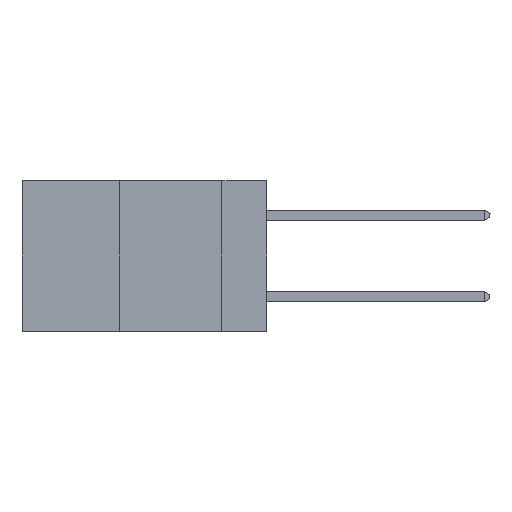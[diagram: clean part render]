
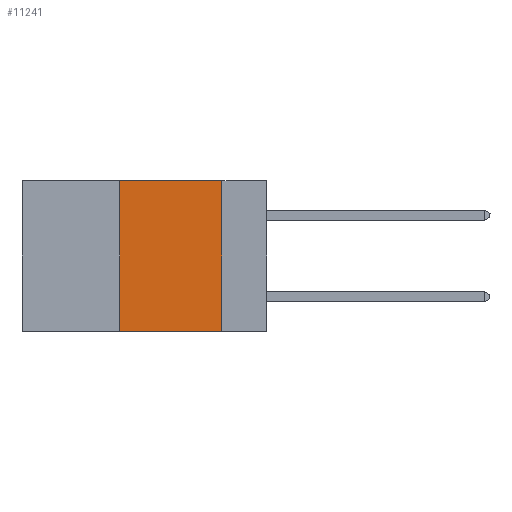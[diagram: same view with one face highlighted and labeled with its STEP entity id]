
A CAD part, left-side view. The second image highlights one B-rep face of the part: STEP entity #11241.
In plain terms, the highlighted planar face has unit normal (-1, 0, 0).
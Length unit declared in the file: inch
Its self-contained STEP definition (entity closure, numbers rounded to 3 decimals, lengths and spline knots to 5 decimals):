
#434 = LINE ( 'NONE', #5004, #16447 ) ;
#929 = EDGE_CURVE ( 'NONE', #17560, #944, #16275, .T. ) ;
#944 = VERTEX_POINT ( 'NONE', #15365 ) ;
#1764 = EDGE_LOOP ( 'NONE', ( #7990, #14603, #2605, #5064 ) ) ;
#2605 = ORIENTED_EDGE ( 'NONE', *, *, #18100, .F. ) ;
#3292 = LINE ( 'NONE', #14685, #11626 ) ;
#3982 = CARTESIAN_POINT ( 'NONE',  ( 0., 0.11, -0.37 ) ) ;
#4413 = AXIS2_PLACEMENT_3D ( 'NONE', #14234, #12730, #7152 ) ;
#5004 = CARTESIAN_POINT ( 'NONE',  ( 0., 0.6, -0.37 ) ) ;
#5064 = ORIENTED_EDGE ( 'NONE', *, *, #7106, .T. ) ;
#5637 = VERTEX_POINT ( 'NONE', #3982 ) ;
#7045 = EDGE_CURVE ( 'NONE', #944, #5637, #3292, .T. ) ;
#7106 = EDGE_CURVE ( 'NONE', #15491, #5637, #434, .T. ) ;
#7152 = DIRECTION ( 'NONE',  ( 0., 0., -1. ) ) ;
#7990 = ORIENTED_EDGE ( 'NONE', *, *, #7045, .F. ) ;
#8467 = FACE_OUTER_BOUND ( 'NONE', #1764, .T. ) ;
#8521 = DIRECTION ( 'NONE',  ( 0., -1., 0. ) ) ;
#9113 = DIRECTION ( 'NONE',  ( 0., -1., 0. ) ) ;
#9523 = CARTESIAN_POINT ( 'NONE',  ( 0., 0.36, -0.37 ) ) ;
#11241 = ADVANCED_FACE ( 'NONE', ( #8467 ), #15675, .F. ) ;
#11626 = VECTOR ( 'NONE', #11979, 39.37008 ) ;
#11979 = DIRECTION ( 'NONE',  ( 0., 0., -1. ) ) ;
#12608 = CARTESIAN_POINT ( 'NONE',  ( 0., 0.6, 0. ) ) ;
#12730 = DIRECTION ( 'NONE',  ( 1., 0., 0. ) ) ;
#13439 = CARTESIAN_POINT ( 'NONE',  ( 0., 0.36, 0. ) ) ;
#14229 = VECTOR ( 'NONE', #16125, 39.37008 ) ;
#14234 = CARTESIAN_POINT ( 'NONE',  ( 0., 0.6, 0. ) ) ;
#14603 = ORIENTED_EDGE ( 'NONE', *, *, #929, .F. ) ;
#14685 = CARTESIAN_POINT ( 'NONE',  ( 0., 0.11, 0. ) ) ;
#14748 = CARTESIAN_POINT ( 'NONE',  ( 0., 0.36, 0. ) ) ;
#15365 = CARTESIAN_POINT ( 'NONE',  ( 0., 0.11, 0. ) ) ;
#15394 = VECTOR ( 'NONE', #8521, 39.37008 ) ;
#15491 = VERTEX_POINT ( 'NONE', #9523 ) ;
#15675 = PLANE ( 'NONE',  #4413 ) ;
#16125 = DIRECTION ( 'NONE',  ( 0., 0., 1. ) ) ;
#16275 = LINE ( 'NONE', #12608, #15394 ) ;
#16447 = VECTOR ( 'NONE', #9113, 39.37008 ) ;
#17560 = VERTEX_POINT ( 'NONE', #14748 ) ;
#17944 = LINE ( 'NONE', #13439, #14229 ) ;
#18100 = EDGE_CURVE ( 'NONE', #15491, #17560, #17944, .T. ) ;
